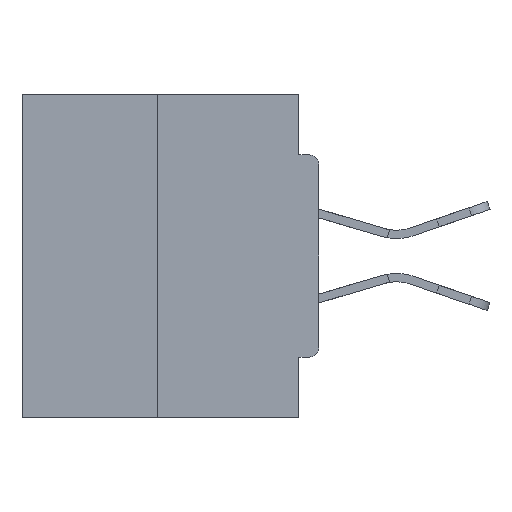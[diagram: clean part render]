
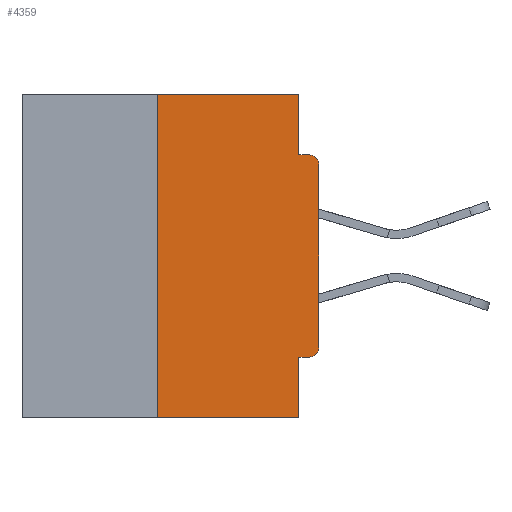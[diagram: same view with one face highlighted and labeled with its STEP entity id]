
A CAD part, left-side view. The second image highlights one B-rep face of the part: STEP entity #4359.
In plain terms, the highlighted planar face has unit normal (-1, 0, 0).
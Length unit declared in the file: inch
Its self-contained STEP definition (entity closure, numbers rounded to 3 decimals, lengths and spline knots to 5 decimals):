
#105 = VECTOR ( 'NONE', #15365, 39.37008 ) ;
#168 = ORIENTED_EDGE ( 'NONE', *, *, #12616, .F. ) ;
#948 = DIRECTION ( 'NONE',  ( 0., 0., 1. ) ) ;
#983 = CARTESIAN_POINT ( 'NONE',  ( 0., 0., -0.4065 ) ) ;
#1393 = VERTEX_POINT ( 'NONE', #35248 ) ;
#1602 = CARTESIAN_POINT ( 'NONE',  ( 0., 0.031, -0.5 ) ) ;
#1762 = CIRCLE ( 'NONE', #35677, 0.015 ) ;
#2251 = DIRECTION ( 'NONE',  ( 0., 0., -1. ) ) ;
#2827 = CARTESIAN_POINT ( 'NONE',  ( 0., 0.25, 0. ) ) ;
#3143 = DIRECTION ( 'NONE',  ( 0., 0., -1. ) ) ;
#3256 = CARTESIAN_POINT ( 'NONE',  ( 0., 0.031, 0. ) ) ;
#4325 = DIRECTION ( 'NONE',  ( 0., -1., 0. ) ) ;
#4359 = ADVANCED_FACE ( 'NONE', ( #24548 ), #5547, .F. ) ;
#4384 = LINE ( 'NONE', #3256, #8998 ) ;
#4541 = LINE ( 'NONE', #2827, #24503 ) ;
#4787 = CARTESIAN_POINT ( 'NONE',  ( 0., 0.015, -0.3915 ) ) ;
#5344 = DIRECTION ( 'NONE',  ( 0., -1., 0. ) ) ;
#5547 = PLANE ( 'NONE',  #28616 ) ;
#6067 = CARTESIAN_POINT ( 'NONE',  ( 0., 0., -0.3915 ) ) ;
#6191 = CARTESIAN_POINT ( 'NONE',  ( 0., 0.031, -0.4065 ) ) ;
#8267 = VECTOR ( 'NONE', #948, 39.37008 ) ;
#8998 = VECTOR ( 'NONE', #3143, 39.37008 ) ;
#9185 = VECTOR ( 'NONE', #4325, 39.37008 ) ;
#10592 = LINE ( 'NONE', #24797, #26902 ) ;
#11114 = ORIENTED_EDGE ( 'NONE', *, *, #30692, .T. ) ;
#11237 = ORIENTED_EDGE ( 'NONE', *, *, #35748, .F. ) ;
#11472 = ORIENTED_EDGE ( 'NONE', *, *, #12905, .T. ) ;
#11589 = CIRCLE ( 'NONE', #22580, 0.015 ) ;
#12094 = DIRECTION ( 'NONE',  ( 0., -1., 0. ) ) ;
#12616 = EDGE_CURVE ( 'NONE', #24612, #36848, #29075, .T. ) ;
#12905 = EDGE_CURVE ( 'NONE', #27383, #26315, #1762, .T. ) ;
#13044 = VERTEX_POINT ( 'NONE', #14335 ) ;
#13082 = ORIENTED_EDGE ( 'NONE', *, *, #14256, .F. ) ;
#13468 = DIRECTION ( 'NONE',  ( -1., 0., 0. ) ) ;
#14256 = EDGE_CURVE ( 'NONE', #1393, #30808, #4541, .T. ) ;
#14335 = CARTESIAN_POINT ( 'NONE',  ( 0., 0.031, -0.0935 ) ) ;
#14597 = ORIENTED_EDGE ( 'NONE', *, *, #27585, .F. ) ;
#15157 = EDGE_CURVE ( 'NONE', #26315, #24630, #27302, .T. ) ;
#15365 = DIRECTION ( 'NONE',  ( 0., 1., 0. ) ) ;
#15893 = CARTESIAN_POINT ( 'NONE',  ( 0., 0.46, 0. ) ) ;
#15981 = EDGE_CURVE ( 'NONE', #24630, #29419, #11589, .T. ) ;
#16596 = ORIENTED_EDGE ( 'NONE', *, *, #15981, .T. ) ;
#16761 = CARTESIAN_POINT ( 'NONE',  ( 0., 0.015, -0.1085 ) ) ;
#17351 = LINE ( 'NONE', #15893, #9185 ) ;
#17719 = DIRECTION ( 'NONE',  ( 0., 0., 1. ) ) ;
#18905 = EDGE_CURVE ( 'NONE', #13044, #29419, #28392, .T. ) ;
#19767 = VECTOR ( 'NONE', #12094, 39.37008 ) ;
#20280 = CARTESIAN_POINT ( 'NONE',  ( 0., 0.46, 0. ) ) ;
#20690 = EDGE_LOOP ( 'NONE', ( #11237, #13082, #11114, #168, #14597, #11472, #34397, #16596, #31753, #29205 ) ) ;
#21227 = CARTESIAN_POINT ( 'NONE',  ( 0., 0.031, 0. ) ) ;
#22580 = AXIS2_PLACEMENT_3D ( 'NONE', #16761, #28155, #34169 ) ;
#22801 = DIRECTION ( 'NONE',  ( 1., 0., 0. ) ) ;
#23723 = CARTESIAN_POINT ( 'NONE',  ( 0., 0.015, -0.4065 ) ) ;
#24503 = VECTOR ( 'NONE', #17719, 39.37008 ) ;
#24548 = FACE_OUTER_BOUND ( 'NONE', #20690, .T. ) ;
#24612 = VERTEX_POINT ( 'NONE', #6191 ) ;
#24630 = VERTEX_POINT ( 'NONE', #29283 ) ;
#24797 = CARTESIAN_POINT ( 'NONE',  ( 0., 0.46, -0.5 ) ) ;
#26315 = VERTEX_POINT ( 'NONE', #6067 ) ;
#26850 = CARTESIAN_POINT ( 'NONE',  ( 0., 0., 0. ) ) ;
#26902 = VECTOR ( 'NONE', #5344, 39.37008 ) ;
#27302 = LINE ( 'NONE', #26850, #8267 ) ;
#27383 = VERTEX_POINT ( 'NONE', #23723 ) ;
#27585 = EDGE_CURVE ( 'NONE', #27383, #24612, #27879, .T. ) ;
#27644 = CARTESIAN_POINT ( 'NONE',  ( 0., 0.25, 0. ) ) ;
#27879 = LINE ( 'NONE', #983, #105 ) ;
#28155 = DIRECTION ( 'NONE',  ( -1., 0., 0. ) ) ;
#28392 = LINE ( 'NONE', #37507, #19767 ) ;
#28616 = AXIS2_PLACEMENT_3D ( 'NONE', #20280, #22801, #31449 ) ;
#29075 = LINE ( 'NONE', #37253, #29972 ) ;
#29205 = ORIENTED_EDGE ( 'NONE', *, *, #36655, .F. ) ;
#29283 = CARTESIAN_POINT ( 'NONE',  ( 0., 0., -0.1085 ) ) ;
#29419 = VERTEX_POINT ( 'NONE', #37308 ) ;
#29972 = VECTOR ( 'NONE', #31514, 39.37008 ) ;
#30692 = EDGE_CURVE ( 'NONE', #1393, #36848, #10592, .T. ) ;
#30808 = VERTEX_POINT ( 'NONE', #27644 ) ;
#31449 = DIRECTION ( 'NONE',  ( 0., 0., -1. ) ) ;
#31514 = DIRECTION ( 'NONE',  ( 0., 0., -1. ) ) ;
#31753 = ORIENTED_EDGE ( 'NONE', *, *, #18905, .F. ) ;
#34169 = DIRECTION ( 'NONE',  ( 0., 0., -1. ) ) ;
#34397 = ORIENTED_EDGE ( 'NONE', *, *, #15157, .T. ) ;
#35248 = CARTESIAN_POINT ( 'NONE',  ( 0., 0.25, -0.5 ) ) ;
#35677 = AXIS2_PLACEMENT_3D ( 'NONE', #4787, #13468, #2251 ) ;
#35748 = EDGE_CURVE ( 'NONE', #30808, #37272, #17351, .T. ) ;
#36655 = EDGE_CURVE ( 'NONE', #37272, #13044, #4384, .T. ) ;
#36848 = VERTEX_POINT ( 'NONE', #1602 ) ;
#37253 = CARTESIAN_POINT ( 'NONE',  ( 0., 0.031, -0.5 ) ) ;
#37272 = VERTEX_POINT ( 'NONE', #21227 ) ;
#37308 = CARTESIAN_POINT ( 'NONE',  ( 0., 0.015, -0.0935 ) ) ;
#37507 = CARTESIAN_POINT ( 'NONE',  ( 0., 0., -0.0935 ) ) ;
